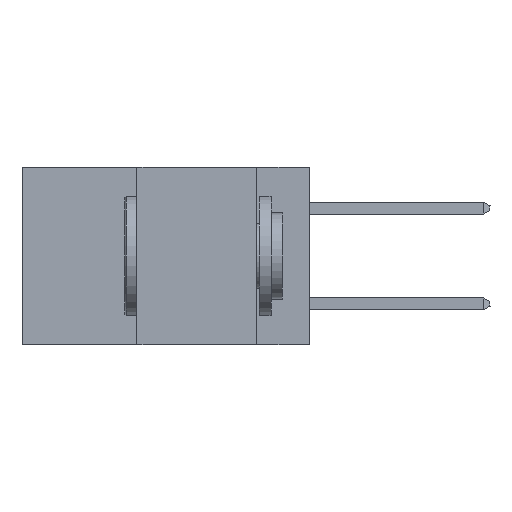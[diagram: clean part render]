
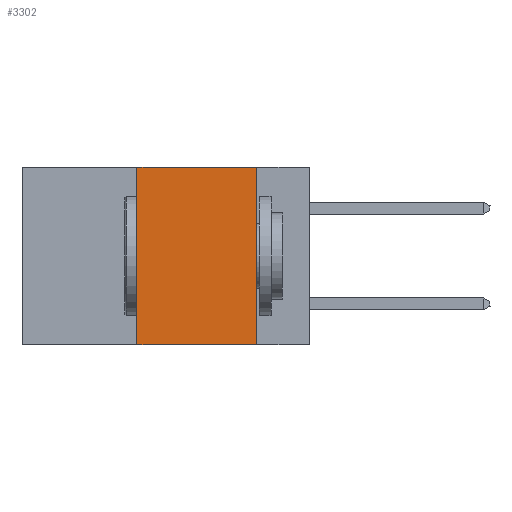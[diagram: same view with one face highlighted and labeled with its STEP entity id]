
A CAD part, left-side view. The second image highlights one B-rep face of the part: STEP entity #3302.
In plain terms, the highlighted planar face has unit normal (-1, 0, 0).
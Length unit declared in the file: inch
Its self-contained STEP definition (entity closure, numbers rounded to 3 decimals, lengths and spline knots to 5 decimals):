
#226 = DIRECTION ( 'NONE',  ( 0., 0., -1. ) ) ;
#824 = DIRECTION ( 'NONE',  ( 0., -1., 0. ) ) ;
#1859 = EDGE_CURVE ( 'NONE', #8013, #4446, #13379, .T. ) ;
#3302 = ADVANCED_FACE ( 'NONE', ( #12348 ), #8467, .F. ) ;
#3360 = ORIENTED_EDGE ( 'NONE', *, *, #15033, .F. ) ;
#3677 = EDGE_CURVE ( 'NONE', #7171, #12430, #12118, .T. ) ;
#4446 = VERTEX_POINT ( 'NONE', #7139 ) ;
#4506 = ORIENTED_EDGE ( 'NONE', *, *, #1859, .T. ) ;
#6458 = EDGE_CURVE ( 'NONE', #8013, #7171, #7034, .T. ) ;
#6647 = CARTESIAN_POINT ( 'NONE',  ( 0., 0.36, 0. ) ) ;
#7030 = DIRECTION ( 'NONE',  ( 1., 0., 0. ) ) ;
#7034 = LINE ( 'NONE', #16358, #14328 ) ;
#7139 = CARTESIAN_POINT ( 'NONE',  ( 0., 0.11, -0.37 ) ) ;
#7171 = VERTEX_POINT ( 'NONE', #6647 ) ;
#7192 = VECTOR ( 'NONE', #9970, 39.37008 ) ;
#7882 = AXIS2_PLACEMENT_3D ( 'NONE', #17780, #7030, #19178 ) ;
#8013 = VERTEX_POINT ( 'NONE', #12756 ) ;
#8338 = CARTESIAN_POINT ( 'NONE',  ( 0., 0.6, -0.37 ) ) ;
#8467 = PLANE ( 'NONE',  #7882 ) ;
#9970 = DIRECTION ( 'NONE',  ( 0., -1., 0. ) ) ;
#10011 = LINE ( 'NONE', #16708, #13536 ) ;
#10310 = VECTOR ( 'NONE', #824, 39.37008 ) ;
#10598 = EDGE_LOOP ( 'NONE', ( #3360, #13883, #16928, #4506 ) ) ;
#12118 = LINE ( 'NONE', #17286, #7192 ) ;
#12348 = FACE_OUTER_BOUND ( 'NONE', #10598, .T. ) ;
#12430 = VERTEX_POINT ( 'NONE', #15938 ) ;
#12756 = CARTESIAN_POINT ( 'NONE',  ( 0., 0.36, -0.37 ) ) ;
#13379 = LINE ( 'NONE', #8338, #10310 ) ;
#13536 = VECTOR ( 'NONE', #226, 39.37008 ) ;
#13787 = DIRECTION ( 'NONE',  ( 0., 0., 1. ) ) ;
#13883 = ORIENTED_EDGE ( 'NONE', *, *, #3677, .F. ) ;
#14328 = VECTOR ( 'NONE', #13787, 39.37008 ) ;
#15033 = EDGE_CURVE ( 'NONE', #12430, #4446, #10011, .T. ) ;
#15938 = CARTESIAN_POINT ( 'NONE',  ( 0., 0.11, 0. ) ) ;
#16358 = CARTESIAN_POINT ( 'NONE',  ( 0., 0.36, 0. ) ) ;
#16708 = CARTESIAN_POINT ( 'NONE',  ( 0., 0.11, 0. ) ) ;
#16928 = ORIENTED_EDGE ( 'NONE', *, *, #6458, .F. ) ;
#17286 = CARTESIAN_POINT ( 'NONE',  ( 0., 0.6, 0. ) ) ;
#17780 = CARTESIAN_POINT ( 'NONE',  ( 0., 0.6, 0. ) ) ;
#19178 = DIRECTION ( 'NONE',  ( 0., 0., -1. ) ) ;
